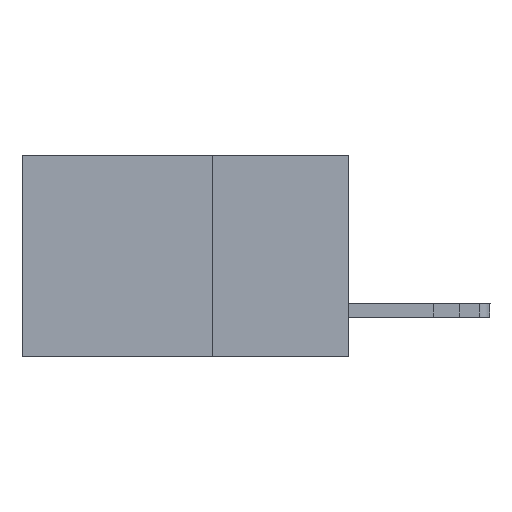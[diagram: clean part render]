
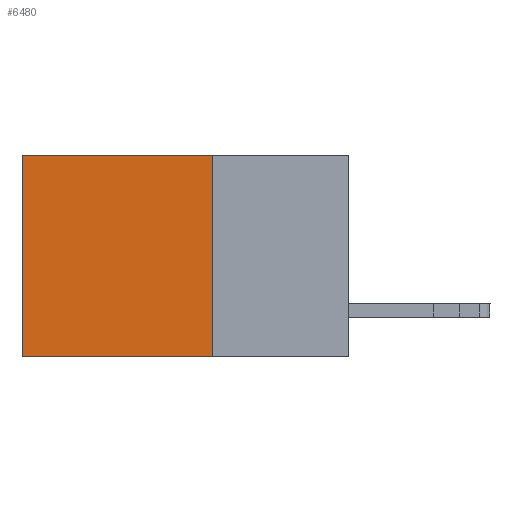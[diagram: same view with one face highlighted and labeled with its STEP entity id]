
A CAD part, left-side view. The second image highlights one B-rep face of the part: STEP entity #6480.
In plain terms, the highlighted planar face has unit normal (-1, 0, 0).
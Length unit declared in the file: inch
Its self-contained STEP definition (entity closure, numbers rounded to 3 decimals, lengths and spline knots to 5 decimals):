
#20 = DIRECTION ( 'NONE',  ( 0., 0., -1. ) ) ;
#123 = CARTESIAN_POINT ( 'NONE',  ( 0.298, 0.25, -0.37 ) ) ;
#162 = EDGE_CURVE ( 'NONE', #2715, #11482, #6001, .T. ) ;
#416 = EDGE_LOOP ( 'NONE', ( #4194, #4658, #10861, #9553 ) ) ;
#690 = CARTESIAN_POINT ( 'NONE',  ( 0.298, 0.6, -0.37 ) ) ;
#1075 = CARTESIAN_POINT ( 'NONE',  ( 0.298, 0.6, 0. ) ) ;
#1549 = DIRECTION ( 'NONE',  ( 0., 0., -1. ) ) ;
#1698 = CARTESIAN_POINT ( 'NONE',  ( 0.298, 0.25, 0. ) ) ;
#2223 = AXIS2_PLACEMENT_3D ( 'NONE', #1698, #11413, #1549 ) ;
#2414 = VERTEX_POINT ( 'NONE', #1075 ) ;
#2715 = VERTEX_POINT ( 'NONE', #5990 ) ;
#2753 = FACE_OUTER_BOUND ( 'NONE', #416, .T. ) ;
#3235 = EDGE_CURVE ( 'NONE', #2414, #7695, #4267, .T. ) ;
#3828 = CARTESIAN_POINT ( 'NONE',  ( 0.298, 0.6, 0. ) ) ;
#3917 = DIRECTION ( 'NONE',  ( 0., 0., -1. ) ) ;
#3962 = CARTESIAN_POINT ( 'NONE',  ( 0.298, 0.25, 0. ) ) ;
#4194 = ORIENTED_EDGE ( 'NONE', *, *, #3235, .T. ) ;
#4239 = VECTOR ( 'NONE', #10061, 39.37008 ) ;
#4267 = LINE ( 'NONE', #3828, #10877 ) ;
#4658 = ORIENTED_EDGE ( 'NONE', *, *, #9615, .F. ) ;
#5990 = CARTESIAN_POINT ( 'NONE',  ( 0.298, 0.25, 0. ) ) ;
#6001 = LINE ( 'NONE', #10648, #10128 ) ;
#6112 = PLANE ( 'NONE',  #2223 ) ;
#6443 = VECTOR ( 'NONE', #10245, 39.37008 ) ;
#6480 = ADVANCED_FACE ( 'NONE', ( #2753 ), #6112, .F. ) ;
#6623 = CARTESIAN_POINT ( 'NONE',  ( 0.298, 0.25, -0.37 ) ) ;
#7695 = VERTEX_POINT ( 'NONE', #690 ) ;
#9553 = ORIENTED_EDGE ( 'NONE', *, *, #10126, .T. ) ;
#9615 = EDGE_CURVE ( 'NONE', #11482, #7695, #10157, .T. ) ;
#10061 = DIRECTION ( 'NONE',  ( 0., 1., 0. ) ) ;
#10126 = EDGE_CURVE ( 'NONE', #2715, #2414, #10168, .T. ) ;
#10128 = VECTOR ( 'NONE', #20, 39.37008 ) ;
#10157 = LINE ( 'NONE', #6623, #6443 ) ;
#10168 = LINE ( 'NONE', #3962, #4239 ) ;
#10245 = DIRECTION ( 'NONE',  ( 0., 1., 0. ) ) ;
#10648 = CARTESIAN_POINT ( 'NONE',  ( 0.298, 0.25, 0. ) ) ;
#10861 = ORIENTED_EDGE ( 'NONE', *, *, #162, .F. ) ;
#10877 = VECTOR ( 'NONE', #3917, 39.37008 ) ;
#11413 = DIRECTION ( 'NONE',  ( 1., 0., 0. ) ) ;
#11482 = VERTEX_POINT ( 'NONE', #123 ) ;
